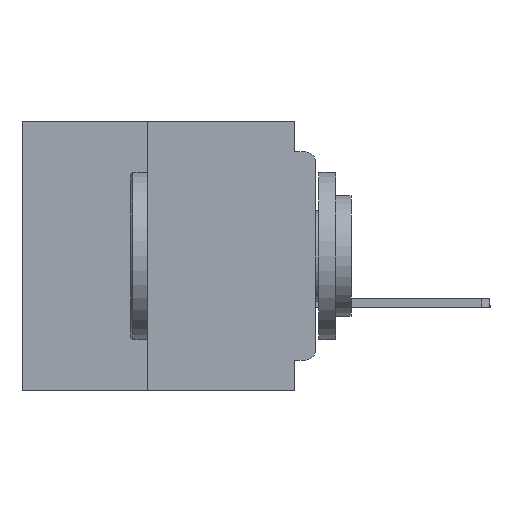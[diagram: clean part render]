
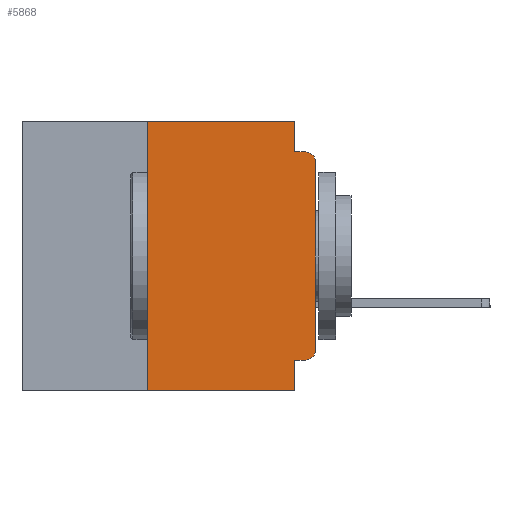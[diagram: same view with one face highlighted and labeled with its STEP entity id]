
A CAD part, left-side view. The second image highlights one B-rep face of the part: STEP entity #5868.
In plain terms, the highlighted planar face has unit normal (-1, 0, 0).
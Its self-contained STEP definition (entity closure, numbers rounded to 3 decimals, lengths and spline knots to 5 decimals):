
#607 = CARTESIAN_POINT ( 'NONE',  ( 0., 0.031, -0.045 ) ) ;
#1875 = EDGE_CURVE ( 'NONE', #47740, #41394, #30897, .T. ) ;
#1885 = DIRECTION ( 'NONE',  ( 0., 0., 1. ) ) ;
#3292 = VERTEX_POINT ( 'NONE', #607 ) ;
#3757 = CARTESIAN_POINT ( 'NONE',  ( 0., 0., 0. ) ) ;
#3907 = LINE ( 'NONE', #58397, #54991 ) ;
#5272 = VERTEX_POINT ( 'NONE', #50108 ) ;
#5744 = CARTESIAN_POINT ( 'NONE',  ( 0., 0.015, -0.06 ) ) ;
#5811 = EDGE_CURVE ( 'NONE', #41394, #37430, #45133, .T. ) ;
#5868 = ADVANCED_FACE ( 'NONE', ( #29052 ), #35951, .F. ) ;
#6179 = VERTEX_POINT ( 'NONE', #8385 ) ;
#7339 = VECTOR ( 'NONE', #54354, 39.37008 ) ;
#7515 = VECTOR ( 'NONE', #63097, 39.37008 ) ;
#8385 = CARTESIAN_POINT ( 'NONE',  ( 0., 0.015, -0.355 ) ) ;
#10093 = EDGE_CURVE ( 'NONE', #6179, #47740, #20619, .T. ) ;
#10838 = DIRECTION ( 'NONE',  ( 0., 0., -1. ) ) ;
#11279 = DIRECTION ( 'NONE',  ( 0., 0., -1. ) ) ;
#11415 = CARTESIAN_POINT ( 'NONE',  ( 0., 0., -0.06 ) ) ;
#14595 = ORIENTED_EDGE ( 'NONE', *, *, #32844, .F. ) ;
#15928 = CARTESIAN_POINT ( 'NONE',  ( 0., 0.25, 0. ) ) ;
#16544 = ORIENTED_EDGE ( 'NONE', *, *, #50218, .F. ) ;
#17118 = LINE ( 'NONE', #58515, #40269 ) ;
#17570 = CARTESIAN_POINT ( 'NONE',  ( 0., 0.25, -0.4 ) ) ;
#18197 = DIRECTION ( 'NONE',  ( 0., -1., 0. ) ) ;
#18767 = LINE ( 'NONE', #17570, #43459 ) ;
#20574 = VERTEX_POINT ( 'NONE', #15928 ) ;
#20619 = CIRCLE ( 'NONE', #48201, 0.015 ) ;
#22166 = LINE ( 'NONE', #33034, #46782 ) ;
#22183 = LINE ( 'NONE', #29960, #7339 ) ;
#22563 = DIRECTION ( 'NONE',  ( 0., 0., 1. ) ) ;
#24347 = ORIENTED_EDGE ( 'NONE', *, *, #5811, .T. ) ;
#24535 = CARTESIAN_POINT ( 'NONE',  ( 0., 0.015, -0.34 ) ) ;
#25215 = VERTEX_POINT ( 'NONE', #34643 ) ;
#25243 = EDGE_CURVE ( 'NONE', #3292, #37430, #22183, .T. ) ;
#25835 = AXIS2_PLACEMENT_3D ( 'NONE', #5744, #40457, #10838 ) ;
#29052 = FACE_OUTER_BOUND ( 'NONE', #35604, .T. ) ;
#29362 = VECTOR ( 'NONE', #1885, 39.37008 ) ;
#29394 = DIRECTION ( 'NONE',  ( 0., -1., 0. ) ) ;
#29554 = DIRECTION ( 'NONE',  ( 0., 0., -1. ) ) ;
#29960 = CARTESIAN_POINT ( 'NONE',  ( 0., 0., -0.045 ) ) ;
#30897 = LINE ( 'NONE', #3757, #29362 ) ;
#32844 = EDGE_CURVE ( 'NONE', #25215, #3292, #3907, .T. ) ;
#33034 = CARTESIAN_POINT ( 'NONE',  ( 0., 0., -0.355 ) ) ;
#34643 = CARTESIAN_POINT ( 'NONE',  ( 0., 0.031, 0. ) ) ;
#35604 = EDGE_LOOP ( 'NONE', ( #44012, #24347, #44491, #14595, #56232, #53602, #38849, #16544, #36309, #48972 ) ) ;
#35951 = PLANE ( 'NONE',  #48848 ) ;
#36309 = ORIENTED_EDGE ( 'NONE', *, *, #36663, .F. ) ;
#36663 = EDGE_CURVE ( 'NONE', #6179, #5272, #22166, .T. ) ;
#37430 = VERTEX_POINT ( 'NONE', #38981 ) ;
#37446 = VERTEX_POINT ( 'NONE', #58708 ) ;
#38151 = DIRECTION ( 'NONE',  ( 0., 1., 0. ) ) ;
#38633 = CARTESIAN_POINT ( 'NONE',  ( 0., 0.031, -0.4 ) ) ;
#38849 = ORIENTED_EDGE ( 'NONE', *, *, #47547, .T. ) ;
#38981 = CARTESIAN_POINT ( 'NONE',  ( 0., 0.015, -0.045 ) ) ;
#39187 = EDGE_CURVE ( 'NONE', #20574, #25215, #17118, .T. ) ;
#40269 = VECTOR ( 'NONE', #29394, 39.37008 ) ;
#40457 = DIRECTION ( 'NONE',  ( -1., 0., 0. ) ) ;
#40879 = DIRECTION ( 'NONE',  ( 1., 0., 0. ) ) ;
#41394 = VERTEX_POINT ( 'NONE', #11415 ) ;
#42530 = VERTEX_POINT ( 'NONE', #54384 ) ;
#42804 = CARTESIAN_POINT ( 'NONE',  ( 0., 0.437, -0.4 ) ) ;
#43459 = VECTOR ( 'NONE', #22563, 39.37008 ) ;
#44012 = ORIENTED_EDGE ( 'NONE', *, *, #1875, .T. ) ;
#44491 = ORIENTED_EDGE ( 'NONE', *, *, #25243, .F. ) ;
#45133 = CIRCLE ( 'NONE', #25835, 0.015 ) ;
#46782 = VECTOR ( 'NONE', #38151, 39.37008 ) ;
#47547 = EDGE_CURVE ( 'NONE', #42530, #37446, #52629, .T. ) ;
#47740 = VERTEX_POINT ( 'NONE', #58829 ) ;
#48201 = AXIS2_PLACEMENT_3D ( 'NONE', #24535, #58868, #29554 ) ;
#48848 = AXIS2_PLACEMENT_3D ( 'NONE', #55472, #40879, #11279 ) ;
#48972 = ORIENTED_EDGE ( 'NONE', *, *, #10093, .T. ) ;
#50108 = CARTESIAN_POINT ( 'NONE',  ( 0., 0.031, -0.355 ) ) ;
#50218 = EDGE_CURVE ( 'NONE', #5272, #37446, #58483, .T. ) ;
#52629 = LINE ( 'NONE', #42804, #64113 ) ;
#53472 = DIRECTION ( 'NONE',  ( 0., 0., -1. ) ) ;
#53602 = ORIENTED_EDGE ( 'NONE', *, *, #62611, .F. ) ;
#54354 = DIRECTION ( 'NONE',  ( 0., -1., 0. ) ) ;
#54384 = CARTESIAN_POINT ( 'NONE',  ( 0., 0.25, -0.4 ) ) ;
#54991 = VECTOR ( 'NONE', #53472, 39.37008 ) ;
#55472 = CARTESIAN_POINT ( 'NONE',  ( 0., 0.437, 0. ) ) ;
#56232 = ORIENTED_EDGE ( 'NONE', *, *, #39187, .F. ) ;
#58397 = CARTESIAN_POINT ( 'NONE',  ( 0., 0.031, 0. ) ) ;
#58483 = LINE ( 'NONE', #38633, #7515 ) ;
#58515 = CARTESIAN_POINT ( 'NONE',  ( 0., 0.437, 0. ) ) ;
#58708 = CARTESIAN_POINT ( 'NONE',  ( 0., 0.031, -0.4 ) ) ;
#58829 = CARTESIAN_POINT ( 'NONE',  ( 0., 0., -0.34 ) ) ;
#58868 = DIRECTION ( 'NONE',  ( -1., 0., 0. ) ) ;
#62611 = EDGE_CURVE ( 'NONE', #42530, #20574, #18767, .T. ) ;
#63097 = DIRECTION ( 'NONE',  ( 0., 0., -1. ) ) ;
#64113 = VECTOR ( 'NONE', #18197, 39.37008 ) ;
